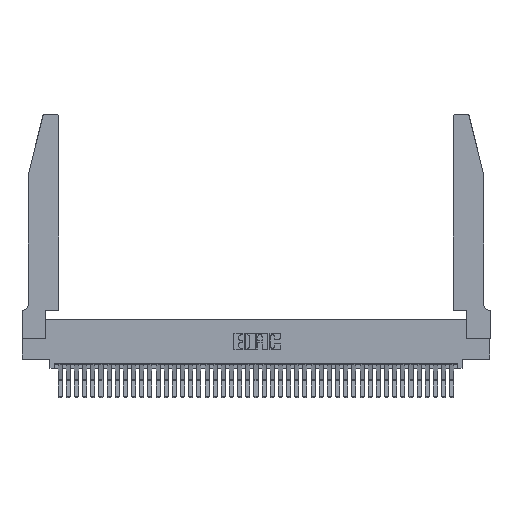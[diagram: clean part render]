
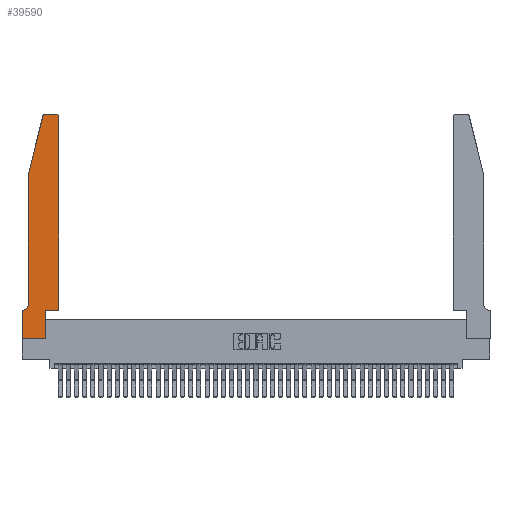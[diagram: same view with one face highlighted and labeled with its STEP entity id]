
A CAD part, top view. The second image highlights one B-rep face of the part: STEP entity #39590.
In plain terms, the highlighted planar face has unit normal (0, 0, 1).
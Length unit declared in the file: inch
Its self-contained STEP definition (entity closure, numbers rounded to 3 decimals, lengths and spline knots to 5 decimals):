
#784 = DIRECTION ( 'NONE',  ( 0., -1., 0. ) ) ;
#1006 = CARTESIAN_POINT ( 'NONE',  ( 0.2865, 0.35, 0.37 ) ) ;
#1444 = DIRECTION ( 'NONE',  ( -1., 0., 0. ) ) ;
#1665 = VERTEX_POINT ( 'NONE', #33173 ) ;
#3013 = DIRECTION ( 'NONE',  ( 0., -1., 0. ) ) ;
#3254 = CARTESIAN_POINT ( 'NONE',  ( 0.0755, 2., 0.37 ) ) ;
#3479 = CARTESIAN_POINT ( 'NONE',  ( 0.284, 2.72, 0.37 ) ) ;
#3597 = CARTESIAN_POINT ( 'NONE',  ( 0.4205, 2.72, 0.37 ) ) ;
#3671 = EDGE_CURVE ( 'NONE', #41085, #15853, #21702, .T. ) ;
#3725 = CARTESIAN_POINT ( 'NONE',  ( 0.4505, 0.35, 0.37 ) ) ;
#3845 = ORIENTED_EDGE ( 'NONE', *, *, #40207, .T. ) ;
#4279 = EDGE_CURVE ( 'NONE', #19977, #1665, #41376, .T. ) ;
#5739 = EDGE_LOOP ( 'NONE', ( #35722, #22316, #19306, #32368, #33523, #16714, #3845, #40092, #34920, #22180, #9738, #15718 ) ) ;
#5890 = CARTESIAN_POINT ( 'NONE',  ( 0.25487, 2.72718, 0.37 ) ) ;
#6338 = CARTESIAN_POINT ( 'NONE',  ( 0.284, 2.75, 0.37 ) ) ;
#6688 = CARTESIAN_POINT ( 'NONE',  ( 0.4505, 0.35, 0.37 ) ) ;
#6737 = EDGE_CURVE ( 'NONE', #15853, #8668, #14243, .T. ) ;
#6887 = DIRECTION ( 'NONE',  ( 0., 0., -1. ) ) ;
#6903 = DIRECTION ( 'NONE',  ( 1., 0., 0. ) ) ;
#7034 = DIRECTION ( 'NONE',  ( 1., 0., 0. ) ) ;
#7216 = CARTESIAN_POINT ( 'NONE',  ( 0.0755, 0.42, 0.37 ) ) ;
#7233 = AXIS2_PLACEMENT_3D ( 'NONE', #26566, #6887, #29779 ) ;
#7574 = VECTOR ( 'NONE', #1444, 39.37008 ) ;
#7836 = CARTESIAN_POINT ( 'NONE',  ( 0., 0.35, 0.37 ) ) ;
#8216 = VERTEX_POINT ( 'NONE', #5890 ) ;
#8668 = VERTEX_POINT ( 'NONE', #7836 ) ;
#8743 = VECTOR ( 'NONE', #30134, 39.37008 ) ;
#9738 = ORIENTED_EDGE ( 'NONE', *, *, #24009, .T. ) ;
#10189 = DIRECTION ( 'NONE',  ( 1., 0., 0. ) ) ;
#10219 = VECTOR ( 'NONE', #784, 39.37008 ) ;
#10239 = VECTOR ( 'NONE', #3013, 39.37008 ) ;
#11006 = EDGE_CURVE ( 'NONE', #39667, #8216, #29932, .T. ) ;
#11069 = CARTESIAN_POINT ( 'NONE',  ( 0.0055, 0.35, 0.37 ) ) ;
#11103 = CARTESIAN_POINT ( 'NONE',  ( 0.0755, 0.35, 0.37 ) ) ;
#11280 = LINE ( 'NONE', #12974, #10239 ) ;
#11804 = VECTOR ( 'NONE', #25358, 39.37008 ) ;
#11881 = CARTESIAN_POINT ( 'NONE',  ( 0.4505, 2.72, 0.37 ) ) ;
#12368 = VERTEX_POINT ( 'NONE', #31754 ) ;
#12588 = DIRECTION ( 'NONE',  ( 0., 0., 1. ) ) ;
#12974 = CARTESIAN_POINT ( 'NONE',  ( 0., 0., 0.37 ) ) ;
#13936 = EDGE_CURVE ( 'NONE', #27448, #19977, #24261, .T. ) ;
#14243 = LINE ( 'NONE', #11103, #38161 ) ;
#14769 = VERTEX_POINT ( 'NONE', #11881 ) ;
#15523 = VECTOR ( 'NONE', #23928, 39.37008 ) ;
#15718 = ORIENTED_EDGE ( 'NONE', *, *, #30907, .T. ) ;
#15853 = VERTEX_POINT ( 'NONE', #11069 ) ;
#16499 = VECTOR ( 'NONE', #10189, 39.37008 ) ;
#16714 = ORIENTED_EDGE ( 'NONE', *, *, #6737, .T. ) ;
#16767 = AXIS2_PLACEMENT_3D ( 'NONE', #3597, #26690, #7034 ) ;
#17518 = LINE ( 'NONE', #29997, #8743 ) ;
#18807 = CARTESIAN_POINT ( 'NONE',  ( 0.0755, 2., 0.37 ) ) ;
#19025 = LINE ( 'NONE', #27107, #10219 ) ;
#19306 = ORIENTED_EDGE ( 'NONE', *, *, #30118, .T. ) ;
#19731 = VERTEX_POINT ( 'NONE', #3254 ) ;
#19977 = VERTEX_POINT ( 'NONE', #1006 ) ;
#21043 = DIRECTION ( 'NONE',  ( -1., 0., 0. ) ) ;
#21387 = CARTESIAN_POINT ( 'NONE',  ( 0.2605, 2.75, 0.37 ) ) ;
#21592 = LINE ( 'NONE', #18807, #11804 ) ;
#21702 = CIRCLE ( 'NONE', #7233, 0.07 ) ;
#22180 = ORIENTED_EDGE ( 'NONE', *, *, #4279, .T. ) ;
#22316 = ORIENTED_EDGE ( 'NONE', *, *, #11006, .T. ) ;
#22371 = CARTESIAN_POINT ( 'NONE',  ( 0., 0.35, 0.37 ) ) ;
#23076 = VECTOR ( 'NONE', #36147, 39.37008 ) ;
#23928 = DIRECTION ( 'NONE',  ( 0., 1., 0. ) ) ;
#24009 = EDGE_CURVE ( 'NONE', #1665, #14769, #32670, .T. ) ;
#24261 = LINE ( 'NONE', #36768, #15523 ) ;
#25358 = DIRECTION ( 'NONE',  ( -0.239, -0.971, 0. ) ) ;
#26566 = CARTESIAN_POINT ( 'NONE',  ( 0.0055, 0.42, 0.37 ) ) ;
#26579 = DIRECTION ( 'NONE',  ( 0., 0., 1. ) ) ;
#26690 = DIRECTION ( 'NONE',  ( 0., 0., 1. ) ) ;
#27012 = VERTEX_POINT ( 'NONE', #28712 ) ;
#27107 = CARTESIAN_POINT ( 'NONE',  ( 0.0755, 2., 0.37 ) ) ;
#27448 = VERTEX_POINT ( 'NONE', #34116 ) ;
#28712 = CARTESIAN_POINT ( 'NONE',  ( 0., 0., 0.37 ) ) ;
#29756 = EDGE_CURVE ( 'NONE', #27012, #27448, #17518, .T. ) ;
#29779 = DIRECTION ( 'NONE',  ( -1., 0., 0. ) ) ;
#29932 = CIRCLE ( 'NONE', #37560, 0.03 ) ;
#29997 = CARTESIAN_POINT ( 'NONE',  ( 0., 0., 0.37 ) ) ;
#30118 = EDGE_CURVE ( 'NONE', #8216, #19731, #21592, .T. ) ;
#30134 = DIRECTION ( 'NONE',  ( 1., 0., 0. ) ) ;
#30907 = EDGE_CURVE ( 'NONE', #14769, #12368, #32720, .T. ) ;
#31051 = EDGE_CURVE ( 'NONE', #19731, #41085, #19025, .T. ) ;
#31754 = CARTESIAN_POINT ( 'NONE',  ( 0.4205, 2.75, 0.37 ) ) ;
#31806 = EDGE_CURVE ( 'NONE', #12368, #39667, #41228, .T. ) ;
#32111 = PLANE ( 'NONE',  #34409 ) ;
#32368 = ORIENTED_EDGE ( 'NONE', *, *, #31051, .T. ) ;
#32670 = LINE ( 'NONE', #6688, #23076 ) ;
#32720 = CIRCLE ( 'NONE', #16767, 0.03 ) ;
#33173 = CARTESIAN_POINT ( 'NONE',  ( 0.4505, 0.35, 0.37 ) ) ;
#33523 = ORIENTED_EDGE ( 'NONE', *, *, #3671, .T. ) ;
#34116 = CARTESIAN_POINT ( 'NONE',  ( 0.2865, 0., 0.37 ) ) ;
#34409 = AXIS2_PLACEMENT_3D ( 'NONE', #22371, #12588, #35411 ) ;
#34920 = ORIENTED_EDGE ( 'NONE', *, *, #13936, .T. ) ;
#35411 = DIRECTION ( 'NONE',  ( 1., 0., 0. ) ) ;
#35722 = ORIENTED_EDGE ( 'NONE', *, *, #31806, .T. ) ;
#36147 = DIRECTION ( 'NONE',  ( 0., 1., 0. ) ) ;
#36768 = CARTESIAN_POINT ( 'NONE',  ( 0.2865, 0.35, 0.37 ) ) ;
#37211 = FACE_OUTER_BOUND ( 'NONE', #5739, .T. ) ;
#37560 = AXIS2_PLACEMENT_3D ( 'NONE', #3479, #26579, #6903 ) ;
#38161 = VECTOR ( 'NONE', #21043, 39.37008 ) ;
#39590 = ADVANCED_FACE ( 'NONE', ( #37211 ), #32111, .T. ) ;
#39667 = VERTEX_POINT ( 'NONE', #6338 ) ;
#40092 = ORIENTED_EDGE ( 'NONE', *, *, #29756, .T. ) ;
#40207 = EDGE_CURVE ( 'NONE', #8668, #27012, #11280, .T. ) ;
#41085 = VERTEX_POINT ( 'NONE', #7216 ) ;
#41228 = LINE ( 'NONE', #21387, #7574 ) ;
#41376 = LINE ( 'NONE', #3725, #16499 ) ;
